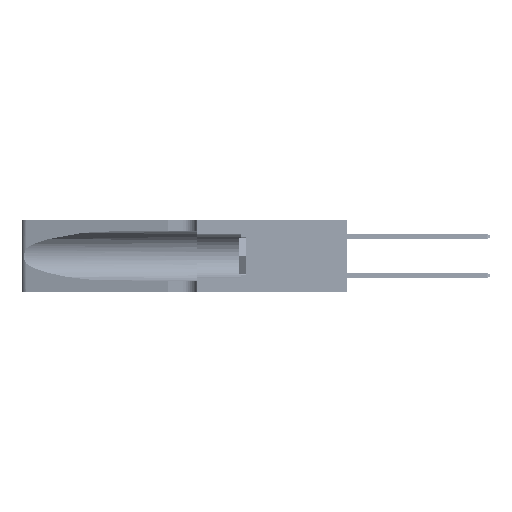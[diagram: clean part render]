
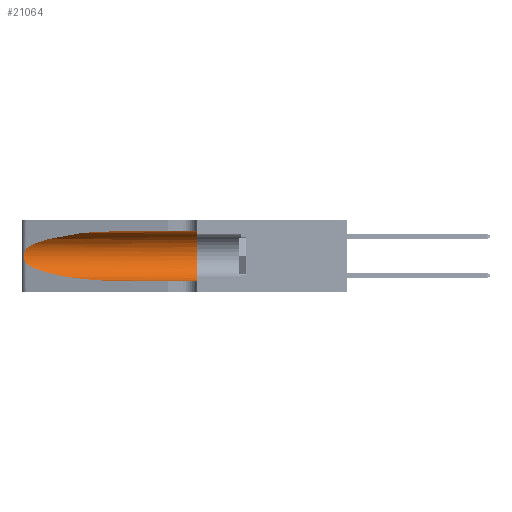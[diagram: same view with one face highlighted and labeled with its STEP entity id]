
A CAD part, left-side view. The second image highlights one B-rep face of the part: STEP entity #21064.
In plain terms, the highlighted cylindrical face has radius 3.308 mm (diameter 6.617 mm), a partial arc.
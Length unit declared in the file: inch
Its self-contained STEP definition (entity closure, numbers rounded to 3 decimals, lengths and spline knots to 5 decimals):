
#91 = CARTESIAN_POINT ( 'NONE',  ( 0.1305, 0.72297, 0.31525 ) ) ;
#296 = CARTESIAN_POINT ( 'NONE',  ( 0.1305, 1.61858, 0.185 ) ) ;
#1245 = CIRCLE ( 'NONE', #2144, 0.13025 ) ;
#1271 = CARTESIAN_POINT ( 'NONE',  ( 0.1305, 0.35, 0.185 ) ) ;
#1885 = VERTEX_POINT ( 'NONE', #26990 ) ;
#2144 = AXIS2_PLACEMENT_3D ( 'NONE', #1271, #28591, #5209 ) ;
#2536 = CARTESIAN_POINT ( 'NONE',  ( 0.26017, 1.23833, 0.17102 ) ) ;
#4920 = CARTESIAN_POINT ( 'NONE',  ( 0.1305, 1.61858, 0.05475 ) ) ;
#5209 = DIRECTION ( 'NONE',  ( 0., 0., 1. ) ) ;
#5866 = VERTEX_POINT ( 'NONE', #6346 ) ;
#6346 = CARTESIAN_POINT ( 'NONE',  ( 0.25487, 1.22718, 0.22369 ) ) ;
#6483 = CARTESIAN_POINT ( 'NONE',  ( 0.25789, 1.23486, 0.15765 ) ) ;
#6961 = EDGE_CURVE ( 'NONE', #29944, #22842, #1245, .T. ) ;
#8009 = CARTESIAN_POINT ( 'NONE',  ( 0.25487, 1.22718, 0.22369 ) ) ;
#8861 = ORIENTED_EDGE ( 'NONE', *, *, #31434, .T. ) ;
#9172 =( BOUNDED_CURVE ( )  B_SPLINE_CURVE ( 3, ( #34431, #15132, #42180, #19066 ),
 .UNSPECIFIED., .F., .T. ) 
 B_SPLINE_CURVE_WITH_KNOTS ( ( 4, 4 ),
 ( 3.44316, 4.71239 ),
 .UNSPECIFIED. ) 
 CURVE ( )  GEOMETRIC_REPRESENTATION_ITEM ( )  RATIONAL_B_SPLINE_CURVE ( ( 1., 0.87, 0.87, 1. ) ) 
 REPRESENTATION_ITEM ( '' )  );
#9865 = EDGE_CURVE ( 'NONE', #25918, #5866, #22016, .T. ) ;
#10408 = CARTESIAN_POINT ( 'NONE',  ( 0.25555, 1.22993, 0.14849 ) ) ;
#15132 = CARTESIAN_POINT ( 'NONE',  ( 0.2373, 1.15595, 0.08982 ) ) ;
#15950 = DIRECTION ( 'NONE',  ( 0., 0., -1. ) ) ;
#17454 = VECTOR ( 'NONE', #43596, 39.37008 ) ;
#18140 = CARTESIAN_POINT ( 'NONE',  ( 0.25787, 1.23484, 0.2124 ) ) ;
#19066 = CARTESIAN_POINT ( 'NONE',  ( 0.1305, 0.72297, 0.05475 ) ) ;
#21064 = ADVANCED_FACE ( 'NONE', ( #38466 ), #47467, .F. ) ;
#22016 =( BOUNDED_CURVE ( )  B_SPLINE_CURVE ( 3, ( #91, #23539, #31329, #8009 ),
 .UNSPECIFIED., .F., .F. ) 
 B_SPLINE_CURVE_WITH_KNOTS ( ( 4, 4 ),
 ( 1.5708, 2.84003 ),
 .UNSPECIFIED. ) 
 CURVE ( )  GEOMETRIC_REPRESENTATION_ITEM ( )  RATIONAL_B_SPLINE_CURVE ( ( 1., 0.87, 0.87, 1. ) ) 
 REPRESENTATION_ITEM ( '' )  );
#22041 = CARTESIAN_POINT ( 'NONE',  ( 0.26018, 1.23835, 0.19895 ) ) ;
#22842 = VERTEX_POINT ( 'NONE', #49264 ) ;
#23539 = CARTESIAN_POINT ( 'NONE',  ( 0.18966, 0.96281, 0.31525 ) ) ;
#24690 = CARTESIAN_POINT ( 'NONE',  ( 0.1305, 0.72297, 0.31525 ) ) ;
#25763 = CARTESIAN_POINT ( 'NONE',  ( 0.25487, 1.22718, 0.22369 ) ) ;
#25918 = VERTEX_POINT ( 'NONE', #24690 ) ;
#25933 = CARTESIAN_POINT ( 'NONE',  ( 0.26075, 1.23896, 0.178 ) ) ;
#26861 = ORIENTED_EDGE ( 'NONE', *, *, #6961, .F. ) ;
#26990 = CARTESIAN_POINT ( 'NONE',  ( 0.25487, 1.22718, 0.14631 ) ) ;
#27339 = DIRECTION ( 'NONE',  ( 0., -1., 0. ) ) ;
#28159 = EDGE_LOOP ( 'NONE', ( #31596, #8861, #46099, #40283, #26861, #37089 ) ) ;
#28591 = DIRECTION ( 'NONE',  ( 0., 1., 0. ) ) ;
#28972 = VERTEX_POINT ( 'NONE', #33368 ) ;
#29668 = CARTESIAN_POINT ( 'NONE',  ( 0.25555, 1.22994, 0.2215 ) ) ;
#29832 = CARTESIAN_POINT ( 'NONE',  ( 0.25856, 1.23593, 0.16098 ) ) ;
#29944 = VERTEX_POINT ( 'NONE', #46875 ) ;
#30980 = EDGE_CURVE ( 'NONE', #25918, #29944, #34706, .T. ) ;
#31329 = CARTESIAN_POINT ( 'NONE',  ( 0.2373, 1.15595, 0.28018 ) ) ;
#31434 = EDGE_CURVE ( 'NONE', #5866, #1885, #36261, .T. ) ;
#31596 = ORIENTED_EDGE ( 'NONE', *, *, #9865, .T. ) ;
#33368 = CARTESIAN_POINT ( 'NONE',  ( 0.1305, 0.72297, 0.05475 ) ) ;
#33507 = VECTOR ( 'NONE', #27339, 39.37008 ) ;
#33703 = CARTESIAN_POINT ( 'NONE',  ( 0.25639, 1.23186, 0.15144 ) ) ;
#34431 = CARTESIAN_POINT ( 'NONE',  ( 0.25487, 1.22718, 0.14631 ) ) ;
#34706 = LINE ( 'NONE', #46507, #33507 ) ;
#36261 = B_SPLINE_CURVE_WITH_KNOTS ( 'NONE', 3,
 ( #25763, #29668, #41293, #18140, #45121, #22041, #48972, #25933, #2536, #29832, #6483, #33703, #10408, #37564 ),
 .UNSPECIFIED., .F., .F.,
 ( 4, 2, 2, 2, 2, 2, 4 ),
 ( 0., 0.00027, 0.00053, 0.00107, 0.0016, 0.00187, 0.00214 ),
 .UNSPECIFIED. ) ;
#37089 = ORIENTED_EDGE ( 'NONE', *, *, #30980, .F. ) ;
#37564 = CARTESIAN_POINT ( 'NONE',  ( 0.25487, 1.22718, 0.14631 ) ) ;
#38466 = FACE_OUTER_BOUND ( 'NONE', #28159, .T. ) ;
#39209 = LINE ( 'NONE', #4920, #17454 ) ;
#40283 = ORIENTED_EDGE ( 'NONE', *, *, #41554, .T. ) ;
#41293 = CARTESIAN_POINT ( 'NONE',  ( 0.25639, 1.23184, 0.21858 ) ) ;
#41554 = EDGE_CURVE ( 'NONE', #28972, #22842, #39209, .T. ) ;
#42180 = CARTESIAN_POINT ( 'NONE',  ( 0.18966, 0.96281, 0.05475 ) ) ;
#43596 = DIRECTION ( 'NONE',  ( 0., -1., 0. ) ) ;
#44132 = EDGE_CURVE ( 'NONE', #1885, #28972, #9172, .T. ) ;
#45121 = CARTESIAN_POINT ( 'NONE',  ( 0.25854, 1.2359, 0.20912 ) ) ;
#45792 = AXIS2_PLACEMENT_3D ( 'NONE', #296, #46829, #15950 ) ;
#46099 = ORIENTED_EDGE ( 'NONE', *, *, #44132, .T. ) ;
#46507 = CARTESIAN_POINT ( 'NONE',  ( 0.1305, 1.61858, 0.31525 ) ) ;
#46829 = DIRECTION ( 'NONE',  ( 0., -1., 0. ) ) ;
#46875 = CARTESIAN_POINT ( 'NONE',  ( 0.1305, 0.35, 0.31525 ) ) ;
#47467 = CYLINDRICAL_SURFACE ( 'NONE', #45792, 0.13025 ) ;
#48972 = CARTESIAN_POINT ( 'NONE',  ( 0.26075, 1.23896, 0.19203 ) ) ;
#49264 = CARTESIAN_POINT ( 'NONE',  ( 0.1305, 0.35, 0.05475 ) ) ;
